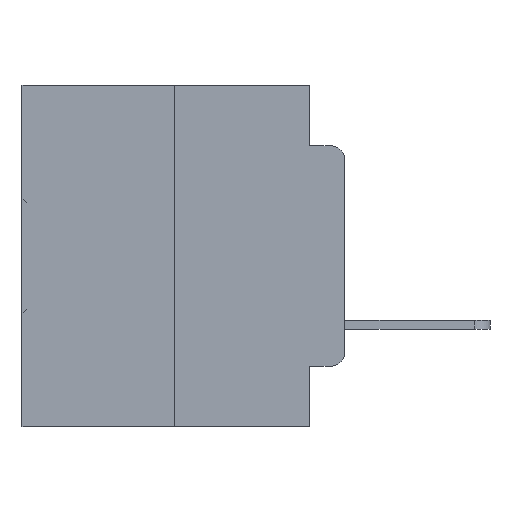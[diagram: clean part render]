
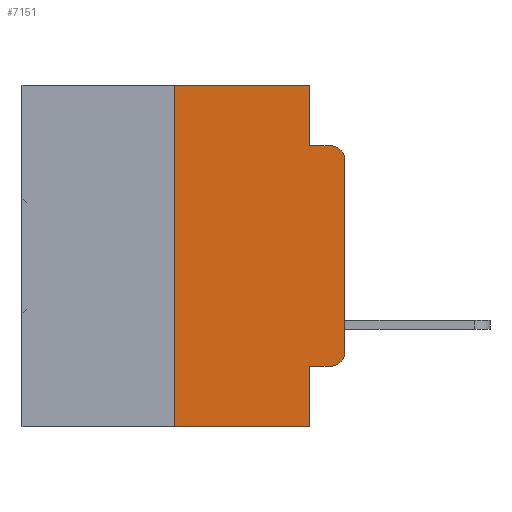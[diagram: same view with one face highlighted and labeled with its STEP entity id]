
A CAD part, left-side view. The second image highlights one B-rep face of the part: STEP entity #7151.
In plain terms, the highlighted planar face has unit normal (-1, 0, 0).
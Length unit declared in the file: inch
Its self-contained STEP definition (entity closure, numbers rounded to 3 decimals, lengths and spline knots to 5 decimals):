
#258 = VECTOR ( 'NONE', #17683, 39.37008 ) ;
#830 = VECTOR ( 'NONE', #23136, 39.37008 ) ;
#839 = VERTEX_POINT ( 'NONE', #19996 ) ;
#854 = ORIENTED_EDGE ( 'NONE', *, *, #4433, .F. ) ;
#1243 = CARTESIAN_POINT ( 'NONE',  ( 0., 0.051, 0. ) ) ;
#1291 = CARTESIAN_POINT ( 'NONE',  ( 0., 0.051, -0.0885 ) ) ;
#1340 = ORIENTED_EDGE ( 'NONE', *, *, #32988, .F. ) ;
#1711 = EDGE_CURVE ( 'NONE', #21242, #21268, #8163, .T. ) ;
#1949 = VERTEX_POINT ( 'NONE', #30468 ) ;
#2371 = CARTESIAN_POINT ( 'NONE',  ( 0., 0.051, 0. ) ) ;
#3629 = VECTOR ( 'NONE', #34510, 39.37008 ) ;
#3679 = EDGE_CURVE ( 'NONE', #21268, #20008, #34595, .T. ) ;
#3986 = ORIENTED_EDGE ( 'NONE', *, *, #5544, .T. ) ;
#4433 = EDGE_CURVE ( 'NONE', #839, #21242, #11277, .T. ) ;
#5544 = EDGE_CURVE ( 'NONE', #21666, #20008, #34816, .T. ) ;
#6234 = EDGE_LOOP ( 'NONE', ( #18608, #3986, #33165, #23471, #854, #1340, #31691, #34088, #33338, #7964 ) ) ;
#6457 = VECTOR ( 'NONE', #11707, 39.37008 ) ;
#6843 = CARTESIAN_POINT ( 'NONE',  ( 0., 0.02, -0.4115 ) ) ;
#6888 = CARTESIAN_POINT ( 'NONE',  ( 0., 0.02, -0.3915 ) ) ;
#7151 = ADVANCED_FACE ( 'NONE', ( #30246 ), #32600, .F. ) ;
#7232 = EDGE_CURVE ( 'NONE', #26766, #26916, #26177, .T. ) ;
#7964 = ORIENTED_EDGE ( 'NONE', *, *, #24285, .T. ) ;
#8163 = LINE ( 'NONE', #2371, #20842 ) ;
#9772 = DIRECTION ( 'NONE',  ( 0., 0., -1. ) ) ;
#9821 = CARTESIAN_POINT ( 'NONE',  ( 0., 0.02, -0.0885 ) ) ;
#10294 = LINE ( 'NONE', #19035, #3629 ) ;
#10397 = VECTOR ( 'NONE', #15571, 39.37008 ) ;
#11277 = LINE ( 'NONE', #28612, #10397 ) ;
#11707 = DIRECTION ( 'NONE',  ( 0., -1., 0. ) ) ;
#11807 = DIRECTION ( 'NONE',  ( 0., 0., -1. ) ) ;
#12393 = DIRECTION ( 'NONE',  ( 0., -1., 0. ) ) ;
#12466 = CARTESIAN_POINT ( 'NONE',  ( 0., 0.25, -0.5 ) ) ;
#13070 = VECTOR ( 'NONE', #14916, 39.37008 ) ;
#13087 = EDGE_CURVE ( 'NONE', #1949, #21666, #10294, .T. ) ;
#13527 = LINE ( 'NONE', #33244, #258 ) ;
#14363 = CARTESIAN_POINT ( 'NONE',  ( 0., 0.051, -0.0885 ) ) ;
#14916 = DIRECTION ( 'NONE',  ( 0., -1., 0. ) ) ;
#15116 = CARTESIAN_POINT ( 'NONE',  ( 0., 0.051, 0. ) ) ;
#15571 = DIRECTION ( 'NONE',  ( 0., -1., 0. ) ) ;
#15707 = LINE ( 'NONE', #1243, #830 ) ;
#16262 = AXIS2_PLACEMENT_3D ( 'NONE', #22298, #27519, #11807 ) ;
#16299 = CARTESIAN_POINT ( 'NONE',  ( 0., 0.02, -0.1085 ) ) ;
#17683 = DIRECTION ( 'NONE',  ( 0., 0., 1. ) ) ;
#18608 = ORIENTED_EDGE ( 'NONE', *, *, #13087, .T. ) ;
#18974 = DIRECTION ( 'NONE',  ( 0., 0., -1. ) ) ;
#19035 = CARTESIAN_POINT ( 'NONE',  ( 0., 0., 0. ) ) ;
#19996 = CARTESIAN_POINT ( 'NONE',  ( 0., 0.25, 0. ) ) ;
#20008 = VERTEX_POINT ( 'NONE', #9821 ) ;
#20033 = CARTESIAN_POINT ( 'NONE',  ( 0., 0.051, -0.4115 ) ) ;
#20842 = VECTOR ( 'NONE', #21518, 39.37008 ) ;
#21242 = VERTEX_POINT ( 'NONE', #15116 ) ;
#21268 = VERTEX_POINT ( 'NONE', #1291 ) ;
#21518 = DIRECTION ( 'NONE',  ( 0., 0., -1. ) ) ;
#21666 = VERTEX_POINT ( 'NONE', #27116 ) ;
#22298 = CARTESIAN_POINT ( 'NONE',  ( 0., 0.473, 0. ) ) ;
#22412 = LINE ( 'NONE', #30666, #29283 ) ;
#23026 = VERTEX_POINT ( 'NONE', #6843 ) ;
#23136 = DIRECTION ( 'NONE',  ( 0., 0., -1. ) ) ;
#23471 = ORIENTED_EDGE ( 'NONE', *, *, #1711, .F. ) ;
#24285 = EDGE_CURVE ( 'NONE', #23026, #1949, #33431, .T. ) ;
#25358 = VERTEX_POINT ( 'NONE', #20033 ) ;
#25625 = DIRECTION ( 'NONE',  ( -1., 0., 0. ) ) ;
#26024 = EDGE_CURVE ( 'NONE', #25358, #23026, #22412, .T. ) ;
#26069 = CARTESIAN_POINT ( 'NONE',  ( 0., 0.051, -0.5 ) ) ;
#26177 = LINE ( 'NONE', #30557, #13070 ) ;
#26766 = VERTEX_POINT ( 'NONE', #12466 ) ;
#26916 = VERTEX_POINT ( 'NONE', #26069 ) ;
#27116 = CARTESIAN_POINT ( 'NONE',  ( 0., 0., -0.1085 ) ) ;
#27519 = DIRECTION ( 'NONE',  ( 1., 0., 0. ) ) ;
#27779 = EDGE_CURVE ( 'NONE', #25358, #26916, #15707, .T. ) ;
#28612 = CARTESIAN_POINT ( 'NONE',  ( 0., 0.473, 0. ) ) ;
#29283 = VECTOR ( 'NONE', #12393, 39.37008 ) ;
#30246 = FACE_OUTER_BOUND ( 'NONE', #6234, .T. ) ;
#30468 = CARTESIAN_POINT ( 'NONE',  ( 0., 0., -0.3915 ) ) ;
#30557 = CARTESIAN_POINT ( 'NONE',  ( 0., 0.473, -0.5 ) ) ;
#30666 = CARTESIAN_POINT ( 'NONE',  ( 0., 0.051, -0.4115 ) ) ;
#31691 = ORIENTED_EDGE ( 'NONE', *, *, #7232, .T. ) ;
#31937 = AXIS2_PLACEMENT_3D ( 'NONE', #16299, #34454, #18974 ) ;
#32600 = PLANE ( 'NONE',  #16262 ) ;
#32988 = EDGE_CURVE ( 'NONE', #26766, #839, #13527, .T. ) ;
#33165 = ORIENTED_EDGE ( 'NONE', *, *, #3679, .F. ) ;
#33244 = CARTESIAN_POINT ( 'NONE',  ( 0., 0.25, 0. ) ) ;
#33338 = ORIENTED_EDGE ( 'NONE', *, *, #26024, .T. ) ;
#33431 = CIRCLE ( 'NONE', #33838, 0.02 ) ;
#33838 = AXIS2_PLACEMENT_3D ( 'NONE', #6888, #25625, #9772 ) ;
#34088 = ORIENTED_EDGE ( 'NONE', *, *, #27779, .F. ) ;
#34454 = DIRECTION ( 'NONE',  ( -1., 0., 0. ) ) ;
#34510 = DIRECTION ( 'NONE',  ( 0., 0., 1. ) ) ;
#34595 = LINE ( 'NONE', #14363, #6457 ) ;
#34816 = CIRCLE ( 'NONE', #31937, 0.02 ) ;
